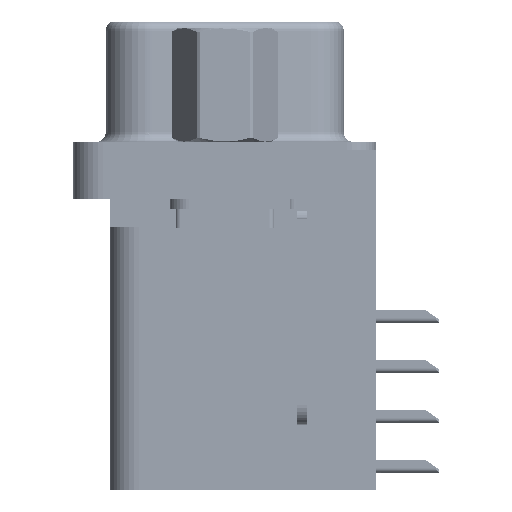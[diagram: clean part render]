
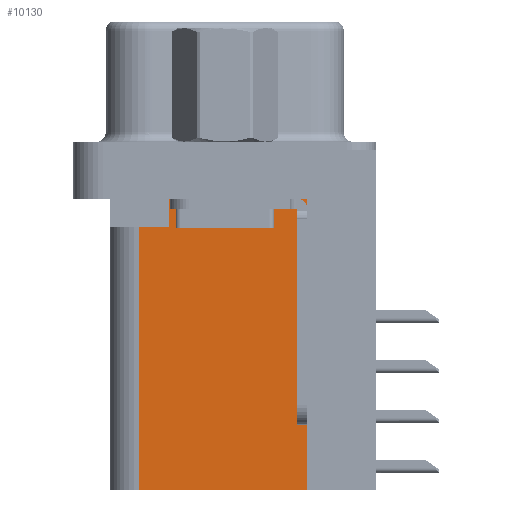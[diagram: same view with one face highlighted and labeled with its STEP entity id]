
A CAD part, left-side view. The second image highlights one B-rep face of the part: STEP entity #10130.
In plain terms, the highlighted planar face has unit normal (-1, 0, 0).
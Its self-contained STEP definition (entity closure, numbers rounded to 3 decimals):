
#1250 = VECTOR ( 'NONE', #34190, 1000. ) ;
#1736 = CARTESIAN_POINT ( 'NONE',  ( 3.75, 2.85, -3.9 ) ) ;
#3176 = EDGE_CURVE ( 'NONE', #25110, #23634, #11081, .T. ) ;
#4080 = PLANE ( 'NONE',  #35961 ) ;
#4895 = LINE ( 'NONE', #43574, #14382 ) ;
#5092 = EDGE_LOOP ( 'NONE', ( #28401, #43488, #44898, #31031, #28291, #30540 ) ) ;
#6380 = VERTEX_POINT ( 'NONE', #1736 ) ;
#7540 = DIRECTION ( 'NONE',  ( 1., 0., 0. ) ) ;
#7671 = DIRECTION ( 'NONE',  ( 0., 1., 0. ) ) ;
#7845 = CARTESIAN_POINT ( 'NONE',  ( 3.75, -4.2, -17.3 ) ) ;
#9065 = CARTESIAN_POINT ( 'NONE',  ( 3.75, 4.35, -3.9 ) ) ;
#9380 = EDGE_CURVE ( 'NONE', #43801, #16193, #14976, .T. ) ;
#9892 = CARTESIAN_POINT ( 'NONE',  ( 3.75, 2.85, -2.5 ) ) ;
#10130 = ADVANCED_FACE ( 'NONE', ( #35237 ), #4080, .F. ) ;
#10395 = CARTESIAN_POINT ( 'NONE',  ( 3.75, 4.35, -17.3 ) ) ;
#11081 = LINE ( 'NONE', #7845, #38063 ) ;
#13602 = CARTESIAN_POINT ( 'NONE',  ( 3.75, -4.2, -17.3 ) ) ;
#13882 = VECTOR ( 'NONE', #45632, 1000. ) ;
#14382 = VECTOR ( 'NONE', #22690, 1000. ) ;
#14976 = LINE ( 'NONE', #35155, #13882 ) ;
#16193 = VERTEX_POINT ( 'NONE', #9892 ) ;
#16705 = CARTESIAN_POINT ( 'NONE',  ( 3.75, 0., -3.9 ) ) ;
#17456 = EDGE_CURVE ( 'NONE', #16193, #6380, #36454, .T. ) ;
#19303 = CARTESIAN_POINT ( 'NONE',  ( 3.75, -4.2, -2.5 ) ) ;
#20265 = LINE ( 'NONE', #16705, #1250 ) ;
#20386 = VECTOR ( 'NONE', #24307, 1000. ) ;
#20730 = EDGE_CURVE ( 'NONE', #6380, #44440, #20265, .T. ) ;
#21814 = CARTESIAN_POINT ( 'NONE',  ( 3.75, -4.2, -17.3 ) ) ;
#22690 = DIRECTION ( 'NONE',  ( 0., 0., 1. ) ) ;
#23634 = VERTEX_POINT ( 'NONE', #10395 ) ;
#24307 = DIRECTION ( 'NONE',  ( 0., 0., 1. ) ) ;
#25110 = VERTEX_POINT ( 'NONE', #43066 ) ;
#28291 = ORIENTED_EDGE ( 'NONE', *, *, #3176, .F. ) ;
#28401 = ORIENTED_EDGE ( 'NONE', *, *, #9380, .T. ) ;
#28455 = EDGE_CURVE ( 'NONE', #23634, #44440, #4895, .T. ) ;
#29701 = LINE ( 'NONE', #13602, #20386 ) ;
#30195 = EDGE_CURVE ( 'NONE', #25110, #43801, #29701, .T. ) ;
#30540 = ORIENTED_EDGE ( 'NONE', *, *, #30195, .T. ) ;
#31031 = ORIENTED_EDGE ( 'NONE', *, *, #28455, .F. ) ;
#31690 = DIRECTION ( 'NONE',  ( 0., 0., -1. ) ) ;
#34190 = DIRECTION ( 'NONE',  ( 0., 1., 0. ) ) ;
#35155 = CARTESIAN_POINT ( 'NONE',  ( 3.75, -4.2, -2.5 ) ) ;
#35237 = FACE_OUTER_BOUND ( 'NONE', #5092, .T. ) ;
#35961 = AXIS2_PLACEMENT_3D ( 'NONE', #21814, #7540, #7671 ) ;
#36454 = LINE ( 'NONE', #38565, #43520 ) ;
#38063 = VECTOR ( 'NONE', #38868, 1000. ) ;
#38565 = CARTESIAN_POINT ( 'NONE',  ( 3.75, 2.85, -3.9 ) ) ;
#38868 = DIRECTION ( 'NONE',  ( 0., 1., 0. ) ) ;
#43066 = CARTESIAN_POINT ( 'NONE',  ( 3.75, -4.2, -17.3 ) ) ;
#43488 = ORIENTED_EDGE ( 'NONE', *, *, #17456, .T. ) ;
#43520 = VECTOR ( 'NONE', #31690, 1000. ) ;
#43574 = CARTESIAN_POINT ( 'NONE',  ( 3.75, 4.35, -17.3 ) ) ;
#43801 = VERTEX_POINT ( 'NONE', #19303 ) ;
#44440 = VERTEX_POINT ( 'NONE', #9065 ) ;
#44898 = ORIENTED_EDGE ( 'NONE', *, *, #20730, .T. ) ;
#45632 = DIRECTION ( 'NONE',  ( 0., 1., 0. ) ) ;
